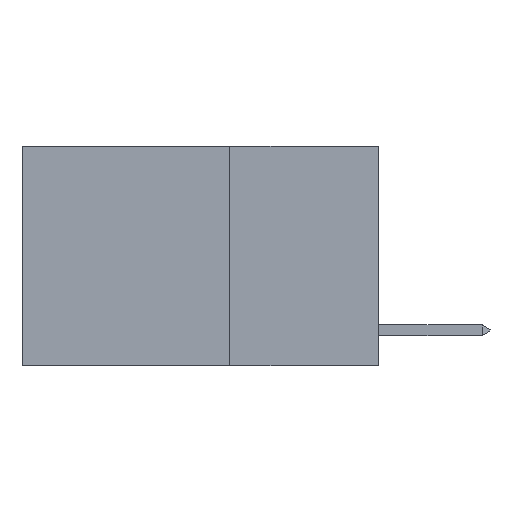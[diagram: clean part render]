
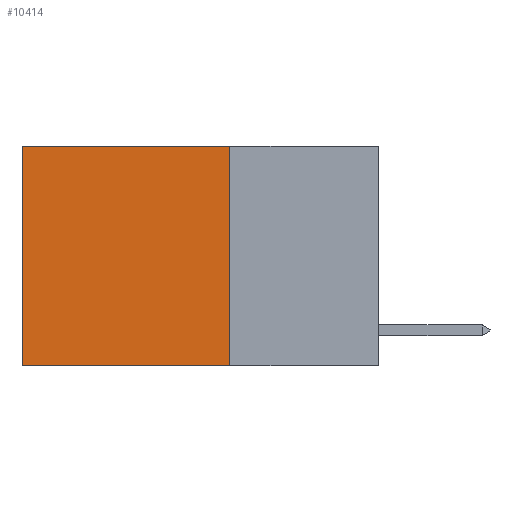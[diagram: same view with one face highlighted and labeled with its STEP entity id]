
A CAD part, left-side view. The second image highlights one B-rep face of the part: STEP entity #10414.
In plain terms, the highlighted planar face has unit normal (-1, 0, 0).
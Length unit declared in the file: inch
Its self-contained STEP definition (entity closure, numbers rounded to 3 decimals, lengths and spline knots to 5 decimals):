
#782 = VECTOR ( 'NONE', #16522, 39.37008 ) ;
#1984 = CARTESIAN_POINT ( 'NONE',  ( 0.2625, 0.25, 0. ) ) ;
#2964 = AXIS2_PLACEMENT_3D ( 'NONE', #18973, #19213, #4405 ) ;
#3705 = EDGE_CURVE ( 'NONE', #20560, #17830, #20970, .T. ) ;
#4405 = DIRECTION ( 'NONE',  ( 0., 0., -1. ) ) ;
#6719 = CARTESIAN_POINT ( 'NONE',  ( 0.2625, 0.6, 0. ) ) ;
#7144 = FACE_OUTER_BOUND ( 'NONE', #16613, .T. ) ;
#7341 = VERTEX_POINT ( 'NONE', #6719 ) ;
#7344 = VECTOR ( 'NONE', #9837, 39.37008 ) ;
#7926 = CARTESIAN_POINT ( 'NONE',  ( 0.2625, 0.6, 0. ) ) ;
#7934 = LINE ( 'NONE', #18210, #782 ) ;
#8228 = EDGE_CURVE ( 'NONE', #7341, #19174, #9091, .T. ) ;
#9031 = CARTESIAN_POINT ( 'NONE',  ( 0.2625, 0.6, -0.37 ) ) ;
#9091 = LINE ( 'NONE', #7926, #23763 ) ;
#9837 = DIRECTION ( 'NONE',  ( 0., 1., 0. ) ) ;
#10414 = ADVANCED_FACE ( 'NONE', ( #7144 ), #22840, .F. ) ;
#11750 = CARTESIAN_POINT ( 'NONE',  ( 0.2625, 0.25, 0. ) ) ;
#12121 = EDGE_CURVE ( 'NONE', #20560, #7341, #15946, .T. ) ;
#15163 = ORIENTED_EDGE ( 'NONE', *, *, #3705, .F. ) ;
#15946 = LINE ( 'NONE', #11750, #7344 ) ;
#16522 = DIRECTION ( 'NONE',  ( 0., 1., 0. ) ) ;
#16613 = EDGE_LOOP ( 'NONE', ( #17674, #19976, #15163, #17358 ) ) ;
#17358 = ORIENTED_EDGE ( 'NONE', *, *, #12121, .T. ) ;
#17674 = ORIENTED_EDGE ( 'NONE', *, *, #8228, .T. ) ;
#17830 = VERTEX_POINT ( 'NONE', #21296 ) ;
#18210 = CARTESIAN_POINT ( 'NONE',  ( 0.2625, 0.25, -0.37 ) ) ;
#18398 = VECTOR ( 'NONE', #21832, 39.37008 ) ;
#18973 = CARTESIAN_POINT ( 'NONE',  ( 0.2625, 0.25, 0. ) ) ;
#19174 = VERTEX_POINT ( 'NONE', #9031 ) ;
#19213 = DIRECTION ( 'NONE',  ( 1., 0., 0. ) ) ;
#19455 = CARTESIAN_POINT ( 'NONE',  ( 0.2625, 0.25, 0. ) ) ;
#19511 = EDGE_CURVE ( 'NONE', #17830, #19174, #7934, .T. ) ;
#19976 = ORIENTED_EDGE ( 'NONE', *, *, #19511, .F. ) ;
#20560 = VERTEX_POINT ( 'NONE', #19455 ) ;
#20566 = DIRECTION ( 'NONE',  ( 0., 0., -1. ) ) ;
#20970 = LINE ( 'NONE', #1984, #18398 ) ;
#21296 = CARTESIAN_POINT ( 'NONE',  ( 0.2625, 0.25, -0.37 ) ) ;
#21832 = DIRECTION ( 'NONE',  ( 0., 0., -1. ) ) ;
#22840 = PLANE ( 'NONE',  #2964 ) ;
#23763 = VECTOR ( 'NONE', #20566, 39.37008 ) ;
